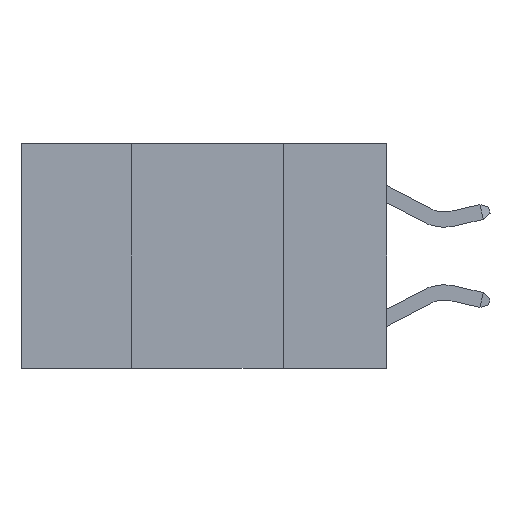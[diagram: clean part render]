
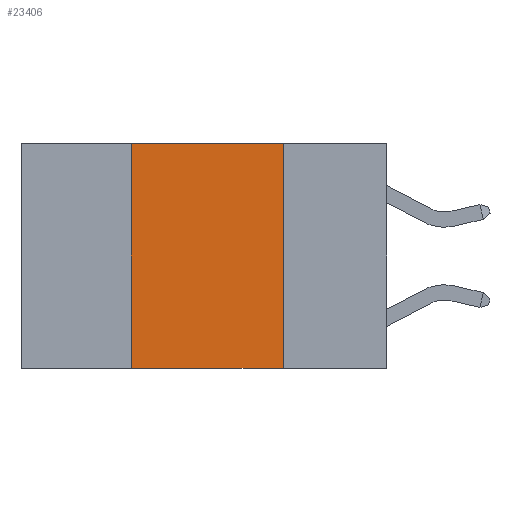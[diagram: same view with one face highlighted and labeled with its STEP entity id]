
A CAD part, left-side view. The second image highlights one B-rep face of the part: STEP entity #23406.
In plain terms, the highlighted planar face has unit normal (-1, 0, 0).
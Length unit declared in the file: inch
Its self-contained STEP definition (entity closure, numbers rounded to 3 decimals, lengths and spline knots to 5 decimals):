
#139 = VECTOR ( 'NONE', #26110, 39.37008 ) ;
#1659 = DIRECTION ( 'NONE',  ( 0., 0., -1. ) ) ;
#2073 = EDGE_LOOP ( 'NONE', ( #28948, #10678, #5775, #18533 ) ) ;
#2195 = CARTESIAN_POINT ( 'NONE',  ( 0., 0.42, 0. ) ) ;
#3440 = AXIS2_PLACEMENT_3D ( 'NONE', #24201, #7574, #24301 ) ;
#3642 = VECTOR ( 'NONE', #7490, 39.37008 ) ;
#5775 = ORIENTED_EDGE ( 'NONE', *, *, #11739, .F. ) ;
#6361 = CARTESIAN_POINT ( 'NONE',  ( 0., 0.17, 0. ) ) ;
#7490 = DIRECTION ( 'NONE',  ( 0., -1., 0. ) ) ;
#7574 = DIRECTION ( 'NONE',  ( 1., 0., 0. ) ) ;
#9293 = LINE ( 'NONE', #21806, #3642 ) ;
#10678 = ORIENTED_EDGE ( 'NONE', *, *, #28227, .F. ) ;
#11030 = CARTESIAN_POINT ( 'NONE',  ( 0., 0.42, 0. ) ) ;
#11739 = EDGE_CURVE ( 'NONE', #17269, #26625, #13898, .T. ) ;
#13288 = LINE ( 'NONE', #6361, #30016 ) ;
#13898 = LINE ( 'NONE', #2195, #26538 ) ;
#15554 = CARTESIAN_POINT ( 'NONE',  ( 0., 0.42, -0.37 ) ) ;
#17269 = VERTEX_POINT ( 'NONE', #15554 ) ;
#18533 = ORIENTED_EDGE ( 'NONE', *, *, #29471, .T. ) ;
#18586 = CARTESIAN_POINT ( 'NONE',  ( 0., 0.17, -0.37 ) ) ;
#18685 = CARTESIAN_POINT ( 'NONE',  ( 0., 0.17, 0. ) ) ;
#18962 = DIRECTION ( 'NONE',  ( 0., 0., 1. ) ) ;
#19992 = LINE ( 'NONE', #30869, #139 ) ;
#21806 = CARTESIAN_POINT ( 'NONE',  ( 0., 0.6, 0. ) ) ;
#21881 = PLANE ( 'NONE',  #3440 ) ;
#23406 = ADVANCED_FACE ( 'NONE', ( #24506 ), #21881, .F. ) ;
#24201 = CARTESIAN_POINT ( 'NONE',  ( 0., 0.6, 0. ) ) ;
#24301 = DIRECTION ( 'NONE',  ( 0., 0., -1. ) ) ;
#24506 = FACE_OUTER_BOUND ( 'NONE', #2073, .T. ) ;
#26110 = DIRECTION ( 'NONE',  ( 0., -1., 0. ) ) ;
#26538 = VECTOR ( 'NONE', #18962, 39.37008 ) ;
#26625 = VERTEX_POINT ( 'NONE', #11030 ) ;
#28001 = VERTEX_POINT ( 'NONE', #18586 ) ;
#28062 = VERTEX_POINT ( 'NONE', #18685 ) ;
#28227 = EDGE_CURVE ( 'NONE', #26625, #28062, #9293, .T. ) ;
#28948 = ORIENTED_EDGE ( 'NONE', *, *, #29299, .F. ) ;
#29299 = EDGE_CURVE ( 'NONE', #28062, #28001, #13288, .T. ) ;
#29471 = EDGE_CURVE ( 'NONE', #17269, #28001, #19992, .T. ) ;
#30016 = VECTOR ( 'NONE', #1659, 39.37008 ) ;
#30869 = CARTESIAN_POINT ( 'NONE',  ( 0., 0.6, -0.37 ) ) ;
